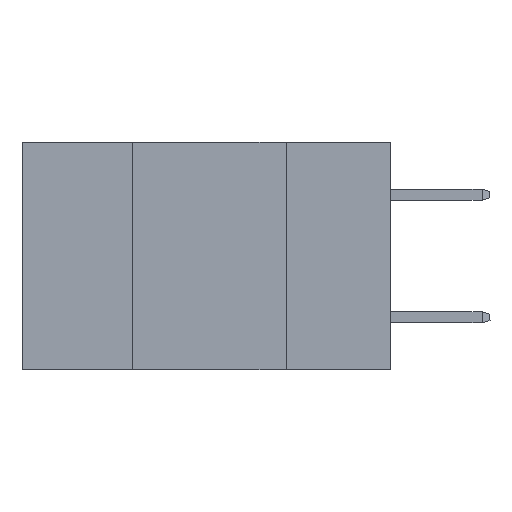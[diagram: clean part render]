
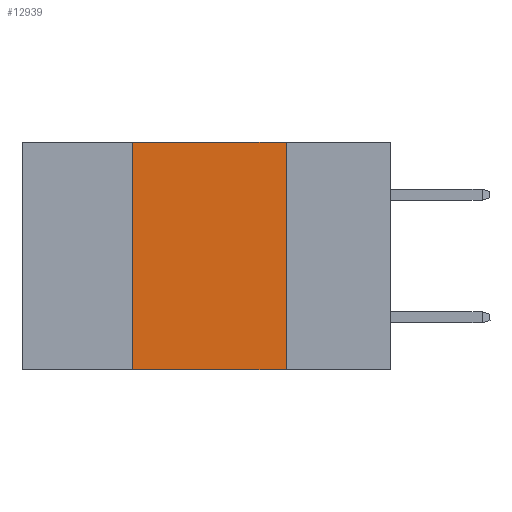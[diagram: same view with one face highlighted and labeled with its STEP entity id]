
A CAD part, left-side view. The second image highlights one B-rep face of the part: STEP entity #12939.
In plain terms, the highlighted planar face has unit normal (-1, 0, 0).
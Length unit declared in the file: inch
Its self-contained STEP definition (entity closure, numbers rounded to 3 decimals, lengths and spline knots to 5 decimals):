
#690 = CARTESIAN_POINT ( 'NONE',  ( 0., 0.42, -0.37 ) ) ;
#1041 = EDGE_LOOP ( 'NONE', ( #14766, #1956, #15954, #8167 ) ) ;
#1182 = EDGE_CURVE ( 'NONE', #10215, #7186, #16690, .T. ) ;
#1956 = ORIENTED_EDGE ( 'NONE', *, *, #9579, .F. ) ;
#2396 = DIRECTION ( 'NONE',  ( 0., -1., 0. ) ) ;
#2771 = VECTOR ( 'NONE', #19554, 39.37008 ) ;
#3806 = VECTOR ( 'NONE', #2396, 39.37008 ) ;
#5084 = DIRECTION ( 'NONE',  ( 1., 0., 0. ) ) ;
#5240 = LINE ( 'NONE', #19250, #8563 ) ;
#5471 = DIRECTION ( 'NONE',  ( 0., -1., 0. ) ) ;
#5545 = CARTESIAN_POINT ( 'NONE',  ( 0., 0.17, 0. ) ) ;
#5713 = CARTESIAN_POINT ( 'NONE',  ( 0., 0.17, -0.37 ) ) ;
#6374 = DIRECTION ( 'NONE',  ( 0., 0., -1. ) ) ;
#6633 = PLANE ( 'NONE',  #17884 ) ;
#6683 = CARTESIAN_POINT ( 'NONE',  ( 0., 0.42, 0. ) ) ;
#7012 = LINE ( 'NONE', #6683, #2771 ) ;
#7186 = VERTEX_POINT ( 'NONE', #5713 ) ;
#8167 = ORIENTED_EDGE ( 'NONE', *, *, #1182, .T. ) ;
#8563 = VECTOR ( 'NONE', #6374, 39.37008 ) ;
#9579 = EDGE_CURVE ( 'NONE', #13700, #19472, #14909, .T. ) ;
#9952 = CARTESIAN_POINT ( 'NONE',  ( 0., 0.6, 0. ) ) ;
#10215 = VERTEX_POINT ( 'NONE', #690 ) ;
#10657 = VECTOR ( 'NONE', #5471, 39.37008 ) ;
#10730 = EDGE_CURVE ( 'NONE', #10215, #13700, #7012, .T. ) ;
#12048 = CARTESIAN_POINT ( 'NONE',  ( 0., 0.6, -0.37 ) ) ;
#12939 = ADVANCED_FACE ( 'NONE', ( #16925 ), #6633, .F. ) ;
#13700 = VERTEX_POINT ( 'NONE', #15040 ) ;
#14766 = ORIENTED_EDGE ( 'NONE', *, *, #20429, .F. ) ;
#14909 = LINE ( 'NONE', #16784, #10657 ) ;
#15040 = CARTESIAN_POINT ( 'NONE',  ( 0., 0.42, 0. ) ) ;
#15954 = ORIENTED_EDGE ( 'NONE', *, *, #10730, .F. ) ;
#16379 = DIRECTION ( 'NONE',  ( 0., 0., -1. ) ) ;
#16690 = LINE ( 'NONE', #12048, #3806 ) ;
#16784 = CARTESIAN_POINT ( 'NONE',  ( 0., 0.6, 0. ) ) ;
#16925 = FACE_OUTER_BOUND ( 'NONE', #1041, .T. ) ;
#17884 = AXIS2_PLACEMENT_3D ( 'NONE', #9952, #5084, #16379 ) ;
#19250 = CARTESIAN_POINT ( 'NONE',  ( 0., 0.17, 0. ) ) ;
#19472 = VERTEX_POINT ( 'NONE', #5545 ) ;
#19554 = DIRECTION ( 'NONE',  ( 0., 0., 1. ) ) ;
#20429 = EDGE_CURVE ( 'NONE', #19472, #7186, #5240, .T. ) ;
